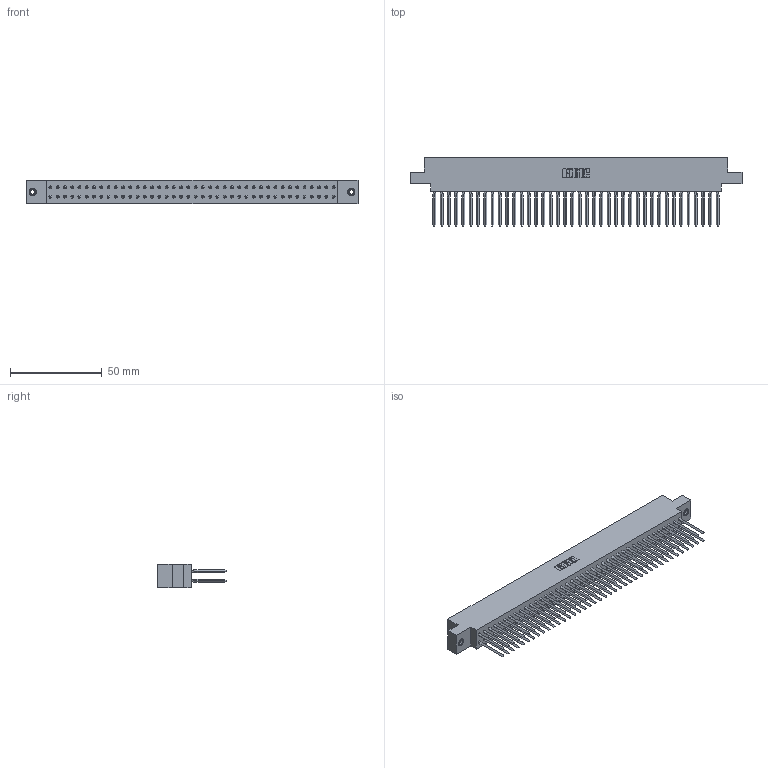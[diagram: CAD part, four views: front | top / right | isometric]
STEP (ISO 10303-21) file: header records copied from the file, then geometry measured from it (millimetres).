
FILE_DESCRIPTION (( 'STEP AP203' ), '1' );
FILE_NAME ('317-080-542-807.STEP', '2020-02-28T09:17:58', ( '' ), ( '' ), 'SwSTEP 2.0', 'SolidWorks 2016', '' );
FILE_SCHEMA (( 'CONFIG_CONTROL_DESIGN' ));
Length unit declared in the file: inch
Products named in the file (4): 317 Part_.156 Dia - TI; 317-080-542-807; 345-250-001_345-250-005-103; 317-290-003_542
Assembly tree (83 placements, depth 2):
  317-080-542-807
    317 Part_.156 Dia - TI
    317-290-003_542  x80
    345-250-001_345-250-005-103  x2
Bounding box: 181.2 x 37.34 x 12.7 mm (x, y, z)
Volume: 29594.8 mm3; surface area: 41126.4 mm2
Topology: 83 solids, 83 shells, 4722 faces, 13211 edges, 8426 vertices
Faces by surface type: plane 3770, cylinder 616, bspline 320, cone 12, torus 4
Entity records: 58302 total; most frequent: CARTESIAN_POINT 10392, ORIENTED_EDGE 10048, DIRECTION 8494, EDGE_CURVE 5024, LINE 4834, VECTOR 4834, VERTEX_POINT 3340, AXIS2_PLACEMENT_3D 1830
